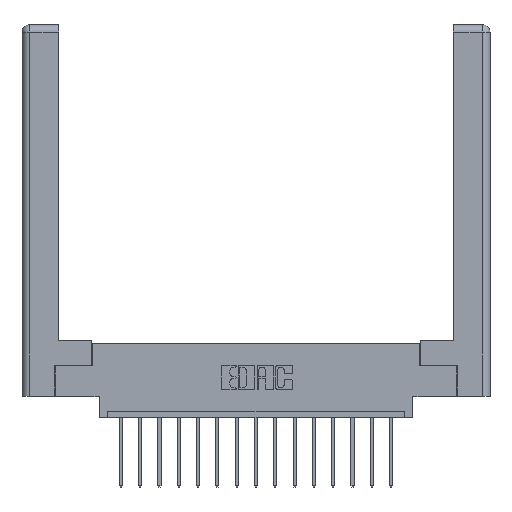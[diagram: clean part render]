
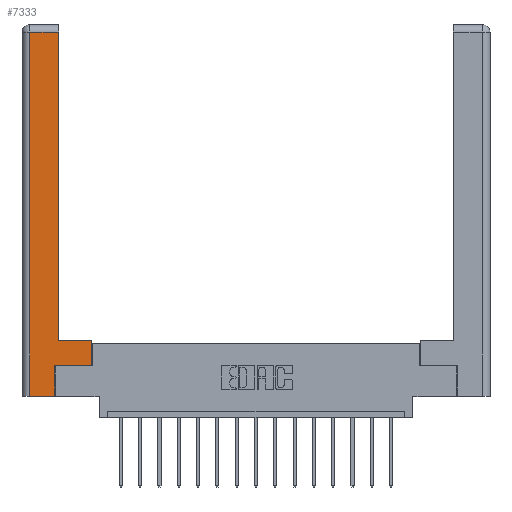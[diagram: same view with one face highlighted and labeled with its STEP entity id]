
A CAD part, top view. The second image highlights one B-rep face of the part: STEP entity #7333.
In plain terms, the highlighted planar face has unit normal (0, 0, 1).
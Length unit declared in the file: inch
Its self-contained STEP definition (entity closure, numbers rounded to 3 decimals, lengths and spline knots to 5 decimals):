
#178 = DIRECTION ( 'NONE',  ( 0., 1., 0. ) ) ;
#654 = VECTOR ( 'NONE', #4178, 39.37008 ) ;
#870 = VERTEX_POINT ( 'NONE', #2976 ) ;
#1026 = DIRECTION ( 'NONE',  ( 0., 0., -1. ) ) ;
#1287 = LINE ( 'NONE', #7306, #11613 ) ;
#1666 = ORIENTED_EDGE ( 'NONE', *, *, #3568, .T. ) ;
#2032 = ORIENTED_EDGE ( 'NONE', *, *, #6990, .T. ) ;
#2320 = EDGE_CURVE ( 'NONE', #14762, #870, #13581, .T. ) ;
#2380 = CARTESIAN_POINT ( 'NONE',  ( 0., 0., 0. ) ) ;
#2443 = CARTESIAN_POINT ( 'NONE',  ( 0.295, 3., 0. ) ) ;
#2670 = CARTESIAN_POINT ( 'NONE',  ( 0.295, 2.94, 0. ) ) ;
#2773 = VERTEX_POINT ( 'NONE', #2670 ) ;
#2976 = CARTESIAN_POINT ( 'NONE',  ( 0.565, 0.45, 0. ) ) ;
#3568 = EDGE_CURVE ( 'NONE', #2773, #5579, #9958, .T. ) ;
#3574 = EDGE_CURVE ( 'NONE', #5579, #4559, #5762, .T. ) ;
#3862 = EDGE_CURVE ( 'NONE', #870, #5327, #12475, .T. ) ;
#3940 = CARTESIAN_POINT ( 'NONE',  ( 0.265, 0., 0. ) ) ;
#4178 = DIRECTION ( 'NONE',  ( -1., 0., 0. ) ) ;
#4235 = EDGE_LOOP ( 'NONE', ( #7096, #1666, #4652, #2032, #12115, #6597, #9353, #10694 ) ) ;
#4559 = VERTEX_POINT ( 'NONE', #10125 ) ;
#4652 = ORIENTED_EDGE ( 'NONE', *, *, #3574, .T. ) ;
#4980 = DIRECTION ( 'NONE',  ( -1., 0., 0. ) ) ;
#5041 = CARTESIAN_POINT ( 'NONE',  ( 0.0615, 2.94, 0. ) ) ;
#5046 = DIRECTION ( 'NONE',  ( -1., 0., 0. ) ) ;
#5327 = VERTEX_POINT ( 'NONE', #5665 ) ;
#5579 = VERTEX_POINT ( 'NONE', #14937 ) ;
#5580 = CARTESIAN_POINT ( 'NONE',  ( 0.265, 0.245, 0. ) ) ;
#5665 = CARTESIAN_POINT ( 'NONE',  ( 0.295, 0.45, 0. ) ) ;
#5762 = LINE ( 'NONE', #10436, #17278 ) ;
#6013 = DIRECTION ( 'NONE',  ( 1., 0., 0. ) ) ;
#6300 = CARTESIAN_POINT ( 'NONE',  ( 0.265, 0., 0. ) ) ;
#6596 = VECTOR ( 'NONE', #4980, 39.37008 ) ;
#6597 = ORIENTED_EDGE ( 'NONE', *, *, #15028, .T. ) ;
#6707 = CARTESIAN_POINT ( 'NONE',  ( 0.265, 0.245, 0. ) ) ;
#6990 = EDGE_CURVE ( 'NONE', #4559, #10268, #10548, .T. ) ;
#7096 = ORIENTED_EDGE ( 'NONE', *, *, #14776, .T. ) ;
#7306 = CARTESIAN_POINT ( 'NONE',  ( 0.565, 0.245, 0. ) ) ;
#7333 = ADVANCED_FACE ( 'NONE', ( #11792 ), #7938, .F. ) ;
#7436 = VECTOR ( 'NONE', #11881, 39.37008 ) ;
#7756 = DIRECTION ( 'NONE',  ( 0., -1., 0. ) ) ;
#7938 = PLANE ( 'NONE',  #11105 ) ;
#8456 = LINE ( 'NONE', #5580, #14672 ) ;
#9280 = VECTOR ( 'NONE', #13354, 39.37008 ) ;
#9353 = ORIENTED_EDGE ( 'NONE', *, *, #2320, .T. ) ;
#9521 = LINE ( 'NONE', #2443, #7436 ) ;
#9958 = LINE ( 'NONE', #5041, #6596 ) ;
#10125 = CARTESIAN_POINT ( 'NONE',  ( 0.0615, 0., 0. ) ) ;
#10268 = VERTEX_POINT ( 'NONE', #6300 ) ;
#10436 = CARTESIAN_POINT ( 'NONE',  ( 0.0615, 0., 0. ) ) ;
#10548 = LINE ( 'NONE', #3940, #9280 ) ;
#10694 = ORIENTED_EDGE ( 'NONE', *, *, #3862, .T. ) ;
#11105 = AXIS2_PLACEMENT_3D ( 'NONE', #2380, #1026, #5046 ) ;
#11172 = CARTESIAN_POINT ( 'NONE',  ( 0.295, 0.45, 0. ) ) ;
#11253 = VERTEX_POINT ( 'NONE', #6707 ) ;
#11613 = VECTOR ( 'NONE', #6013, 39.37008 ) ;
#11645 = CARTESIAN_POINT ( 'NONE',  ( 0.565, 0.245, 0. ) ) ;
#11792 = FACE_OUTER_BOUND ( 'NONE', #4235, .T. ) ;
#11881 = DIRECTION ( 'NONE',  ( 0., 1., 0. ) ) ;
#12115 = ORIENTED_EDGE ( 'NONE', *, *, #12552, .T. ) ;
#12475 = LINE ( 'NONE', #11172, #654 ) ;
#12552 = EDGE_CURVE ( 'NONE', #10268, #11253, #8456, .T. ) ;
#13354 = DIRECTION ( 'NONE',  ( 1., 0., 0. ) ) ;
#13581 = LINE ( 'NONE', #15509, #16740 ) ;
#14672 = VECTOR ( 'NONE', #178, 39.37008 ) ;
#14762 = VERTEX_POINT ( 'NONE', #11645 ) ;
#14776 = EDGE_CURVE ( 'NONE', #5327, #2773, #9521, .T. ) ;
#14937 = CARTESIAN_POINT ( 'NONE',  ( 0.0615, 2.94, 0. ) ) ;
#15028 = EDGE_CURVE ( 'NONE', #11253, #14762, #1287, .T. ) ;
#15509 = CARTESIAN_POINT ( 'NONE',  ( 0.565, 0.45, 0. ) ) ;
#16375 = DIRECTION ( 'NONE',  ( 0., 1., 0. ) ) ;
#16740 = VECTOR ( 'NONE', #16375, 39.37008 ) ;
#17278 = VECTOR ( 'NONE', #7756, 39.37008 ) ;
